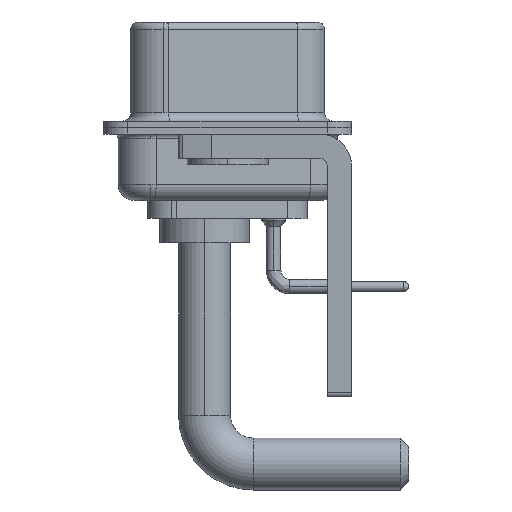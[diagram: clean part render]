
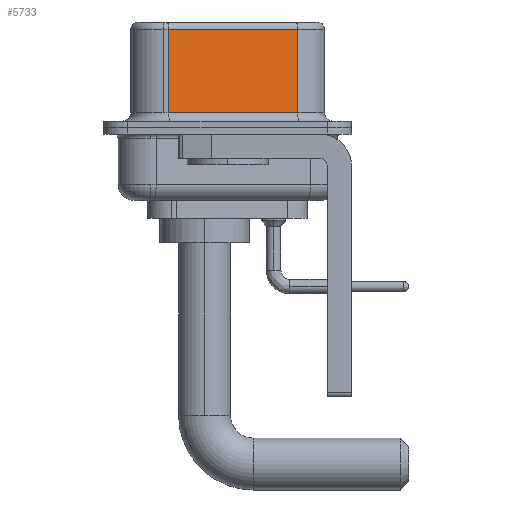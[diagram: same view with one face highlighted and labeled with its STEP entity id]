
A CAD part, left-side view. The second image highlights one B-rep face of the part: STEP entity #5733.
In plain terms, the highlighted planar face has unit normal (-0.985, -0.174, 0).
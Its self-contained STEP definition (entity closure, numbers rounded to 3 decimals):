
#31 = ORIENTED_EDGE ( 'NONE', *, *, #19185, .T. ) ;
#729 = DIRECTION ( 'NONE',  ( 0., 0., -1. ) ) ;
#967 = CARTESIAN_POINT ( 'NONE',  ( 3.73, 3.628, 6.02 ) ) ;
#2235 = CARTESIAN_POINT ( 'NONE',  ( 3.73, 3.628, 0.9 ) ) ;
#2370 = LINE ( 'NONE', #4228, #8834 ) ;
#3041 = DIRECTION ( 'NONE',  ( 0., 0., -1. ) ) ;
#4228 = CARTESIAN_POINT ( 'NONE',  ( 5.132, -4.322, 6.52 ) ) ;
#5151 = DIRECTION ( 'NONE',  ( 0.174, -0.985, 0. ) ) ;
#5733 = ADVANCED_FACE ( 'NONE', ( #8076 ), #15814, .F. ) ;
#6543 = VERTEX_POINT ( 'NONE', #22489 ) ;
#7647 = VERTEX_POINT ( 'NONE', #2235 ) ;
#8076 = FACE_OUTER_BOUND ( 'NONE', #17532, .T. ) ;
#8834 = VECTOR ( 'NONE', #729, 1000. ) ;
#9155 = VECTOR ( 'NONE', #3041, 1000. ) ;
#9450 = VECTOR ( 'NONE', #14493, 1000. ) ;
#9884 = AXIS2_PLACEMENT_3D ( 'NONE', #19172, #11930, #13924 ) ;
#10215 = EDGE_CURVE ( 'NONE', #24587, #6543, #2370, .T. ) ;
#11930 = DIRECTION ( 'NONE',  ( 0.985, 0.174, 0. ) ) ;
#13924 = DIRECTION ( 'NONE',  ( -0.174, 0.985, 0. ) ) ;
#14261 = CARTESIAN_POINT ( 'NONE',  ( 5.132, -4.322, 6.02 ) ) ;
#14493 = DIRECTION ( 'NONE',  ( -0.174, 0.985, 0. ) ) ;
#14641 = ORIENTED_EDGE ( 'NONE', *, *, #10215, .F. ) ;
#15667 = ORIENTED_EDGE ( 'NONE', *, *, #16522, .T. ) ;
#15814 = PLANE ( 'NONE',  #9884 ) ;
#16522 = EDGE_CURVE ( 'NONE', #24587, #22579, #22347, .T. ) ;
#17365 = EDGE_CURVE ( 'NONE', #7647, #6543, #22233, .T. ) ;
#17532 = EDGE_LOOP ( 'NONE', ( #14641, #15667, #31, #17882 ) ) ;
#17882 = ORIENTED_EDGE ( 'NONE', *, *, #17365, .T. ) ;
#17902 = LINE ( 'NONE', #20119, #9155 ) ;
#18587 = VECTOR ( 'NONE', #5151, 1000. ) ;
#18884 = CARTESIAN_POINT ( 'NONE',  ( 5.132, -4.322, 0.9 ) ) ;
#19172 = CARTESIAN_POINT ( 'NONE',  ( 5.132, -4.322, 6.52 ) ) ;
#19185 = EDGE_CURVE ( 'NONE', #22579, #7647, #17902, .T. ) ;
#20119 = CARTESIAN_POINT ( 'NONE',  ( 3.73, 3.628, 6.52 ) ) ;
#22233 = LINE ( 'NONE', #18884, #18587 ) ;
#22347 = LINE ( 'NONE', #14261, #9450 ) ;
#22357 = CARTESIAN_POINT ( 'NONE',  ( 5.132, -4.322, 6.02 ) ) ;
#22489 = CARTESIAN_POINT ( 'NONE',  ( 5.132, -4.322, 0.9 ) ) ;
#22579 = VERTEX_POINT ( 'NONE', #967 ) ;
#24587 = VERTEX_POINT ( 'NONE', #22357 ) ;
